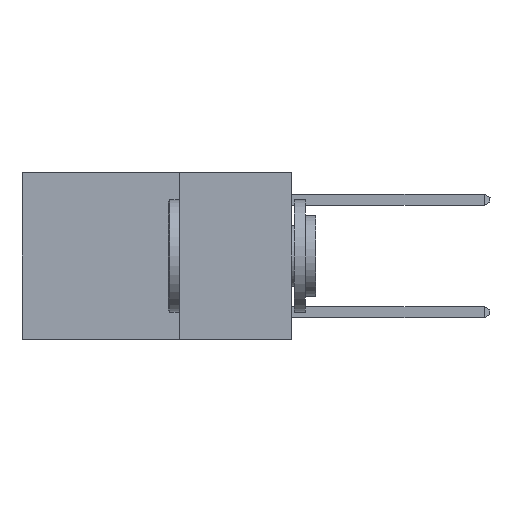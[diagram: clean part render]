
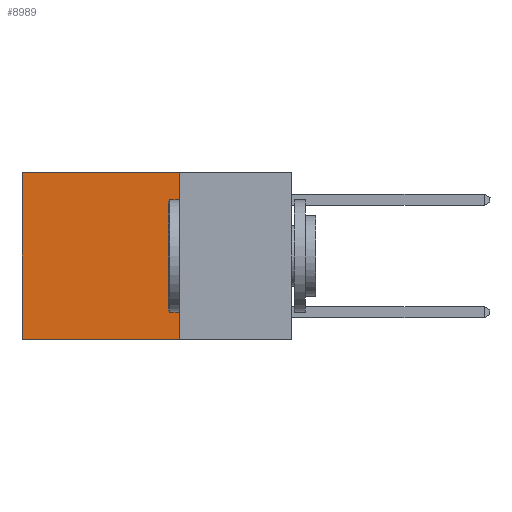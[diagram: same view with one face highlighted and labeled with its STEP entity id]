
A CAD part, left-side view. The second image highlights one B-rep face of the part: STEP entity #8989.
In plain terms, the highlighted planar face has unit normal (-1, 0, 0).
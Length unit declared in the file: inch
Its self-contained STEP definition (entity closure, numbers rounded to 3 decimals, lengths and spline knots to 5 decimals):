
#644 = EDGE_CURVE ( 'NONE', #12626, #14433, #6701, .T. ) ;
#957 = ORIENTED_EDGE ( 'NONE', *, *, #644, .F. ) ;
#1263 = EDGE_LOOP ( 'NONE', ( #8247, #957, #2232, #14490 ) ) ;
#1334 = LINE ( 'NONE', #15172, #12104 ) ;
#2232 = ORIENTED_EDGE ( 'NONE', *, *, #15509, .F. ) ;
#2292 = EDGE_CURVE ( 'NONE', #6580, #3322, #9114, .T. ) ;
#2457 = CARTESIAN_POINT ( 'NONE',  ( 0.2625, 0.25, 0. ) ) ;
#3322 = VERTEX_POINT ( 'NONE', #9138 ) ;
#5564 = DIRECTION ( 'NONE',  ( 0., 1., 0. ) ) ;
#6580 = VERTEX_POINT ( 'NONE', #12850 ) ;
#6611 = DIRECTION ( 'NONE',  ( 0., 0., -1. ) ) ;
#6686 = VECTOR ( 'NONE', #13977, 39.37008 ) ;
#6701 = LINE ( 'NONE', #9493, #13548 ) ;
#6790 = DIRECTION ( 'NONE',  ( 0., 1., 0. ) ) ;
#7348 = EDGE_CURVE ( 'NONE', #3322, #14433, #1334, .T. ) ;
#8247 = ORIENTED_EDGE ( 'NONE', *, *, #7348, .T. ) ;
#8874 = VECTOR ( 'NONE', #6790, 39.37008 ) ;
#8989 = ADVANCED_FACE ( 'NONE', ( #12168 ), #12244, .F. ) ;
#9114 = LINE ( 'NONE', #10416, #8874 ) ;
#9138 = CARTESIAN_POINT ( 'NONE',  ( 0.2625, 0.6, 0. ) ) ;
#9262 = AXIS2_PLACEMENT_3D ( 'NONE', #2457, #9744, #14757 ) ;
#9493 = CARTESIAN_POINT ( 'NONE',  ( 0.2625, 0.25, -0.37 ) ) ;
#9744 = DIRECTION ( 'NONE',  ( 1., 0., 0. ) ) ;
#10416 = CARTESIAN_POINT ( 'NONE',  ( 0.2625, 0.25, 0. ) ) ;
#11144 = CARTESIAN_POINT ( 'NONE',  ( 0.2625, 0.6, -0.37 ) ) ;
#11301 = CARTESIAN_POINT ( 'NONE',  ( 0.2625, 0.25, 0. ) ) ;
#12104 = VECTOR ( 'NONE', #6611, 39.37008 ) ;
#12168 = FACE_OUTER_BOUND ( 'NONE', #1263, .T. ) ;
#12244 = PLANE ( 'NONE',  #9262 ) ;
#12465 = CARTESIAN_POINT ( 'NONE',  ( 0.2625, 0.25, -0.37 ) ) ;
#12611 = LINE ( 'NONE', #11301, #6686 ) ;
#12626 = VERTEX_POINT ( 'NONE', #12465 ) ;
#12850 = CARTESIAN_POINT ( 'NONE',  ( 0.2625, 0.25, 0. ) ) ;
#13548 = VECTOR ( 'NONE', #5564, 39.37008 ) ;
#13977 = DIRECTION ( 'NONE',  ( 0., 0., -1. ) ) ;
#14433 = VERTEX_POINT ( 'NONE', #11144 ) ;
#14490 = ORIENTED_EDGE ( 'NONE', *, *, #2292, .T. ) ;
#14757 = DIRECTION ( 'NONE',  ( 0., 0., -1. ) ) ;
#15172 = CARTESIAN_POINT ( 'NONE',  ( 0.2625, 0.6, 0. ) ) ;
#15509 = EDGE_CURVE ( 'NONE', #6580, #12626, #12611, .T. ) ;
